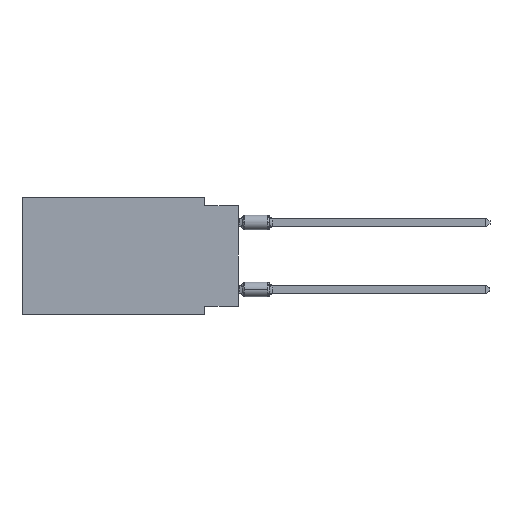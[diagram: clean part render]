
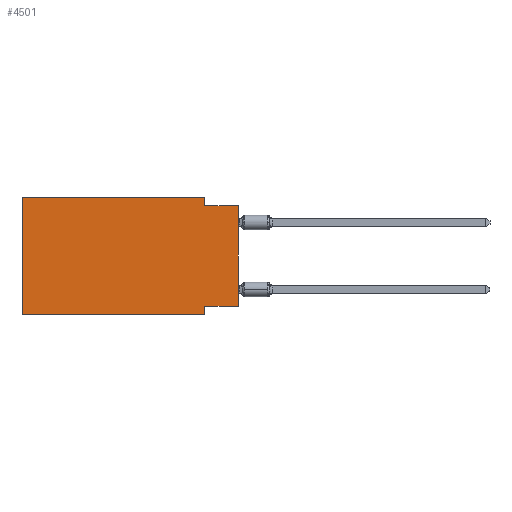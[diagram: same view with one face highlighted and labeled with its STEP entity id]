
A CAD part, left-side view. The second image highlights one B-rep face of the part: STEP entity #4501.
In plain terms, the highlighted planar face has unit normal (-1, 0, 0).
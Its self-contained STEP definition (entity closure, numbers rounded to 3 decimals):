
#44 = VECTOR ( 'NONE', #213, 1000. ) ;
#213 = DIRECTION ( 'NONE',  ( 0., 0., -1. ) ) ;
#262 = DIRECTION ( 'NONE',  ( 0., -1., 0. ) ) ;
#1433 = VECTOR ( 'NONE', #262, 1000. ) ;
#1509 = LINE ( 'NONE', #4698, #1433 ) ;
#1945 = VERTEX_POINT ( 'NONE', #4365 ) ;
#2115 = CARTESIAN_POINT ( 'NONE',  ( 0., 16.383, 0. ) ) ;
#2302 = CARTESIAN_POINT ( 'NONE',  ( 0., 0., -8.255 ) ) ;
#2390 = CARTESIAN_POINT ( 'NONE',  ( 0., 0., -8.255 ) ) ;
#2493 = DIRECTION ( 'NONE',  ( 0., -1., 0. ) ) ;
#2716 = DIRECTION ( 'NONE',  ( 0., 0., -1. ) ) ;
#3091 = DIRECTION ( 'NONE',  ( 0., 0., 1. ) ) ;
#3220 = LINE ( 'NONE', #2390, #13287 ) ;
#3222 = EDGE_CURVE ( 'NONE', #7645, #12915, #7811, .T. ) ;
#3392 = CARTESIAN_POINT ( 'NONE',  ( 0., 16.383, 0. ) ) ;
#3419 = VECTOR ( 'NONE', #2716, 1000. ) ;
#3445 = EDGE_CURVE ( 'NONE', #5342, #11242, #9106, .T. ) ;
#4265 = DIRECTION ( 'NONE',  ( 0., 1., 0. ) ) ;
#4323 = LINE ( 'NONE', #7344, #7355 ) ;
#4365 = CARTESIAN_POINT ( 'NONE',  ( 0., 2.54, 0. ) ) ;
#4501 = ADVANCED_FACE ( 'NONE', ( #11886 ), #9807, .F. ) ;
#4565 = VERTEX_POINT ( 'NONE', #12417 ) ;
#4698 = CARTESIAN_POINT ( 'NONE',  ( 0., 0., -0.635 ) ) ;
#5342 = VERTEX_POINT ( 'NONE', #2302 ) ;
#5819 = EDGE_CURVE ( 'NONE', #5342, #7645, #3220, .T. ) ;
#6143 = ORIENTED_EDGE ( 'NONE', *, *, #3222, .F. ) ;
#6199 = VERTEX_POINT ( 'NONE', #9543 ) ;
#6207 = EDGE_CURVE ( 'NONE', #4565, #12915, #4323, .T. ) ;
#6548 = EDGE_CURVE ( 'NONE', #1945, #13433, #13327, .T. ) ;
#6882 = ORIENTED_EDGE ( 'NONE', *, *, #6207, .T. ) ;
#7131 = EDGE_CURVE ( 'NONE', #13433, #11242, #1509, .T. ) ;
#7344 = CARTESIAN_POINT ( 'NONE',  ( 0., 16.383, -8.89 ) ) ;
#7355 = VECTOR ( 'NONE', #8504, 1000. ) ;
#7645 = VERTEX_POINT ( 'NONE', #11917 ) ;
#7674 = CARTESIAN_POINT ( 'NONE',  ( 0., 16.383, 0. ) ) ;
#7749 = DIRECTION ( 'NONE',  ( 1., 0., 0. ) ) ;
#7811 = LINE ( 'NONE', #11882, #44 ) ;
#8504 = DIRECTION ( 'NONE',  ( 0., -1., 0. ) ) ;
#8755 = EDGE_CURVE ( 'NONE', #4565, #6199, #11571, .T. ) ;
#8764 = DIRECTION ( 'NONE',  ( 0., 0., -1. ) ) ;
#8777 = VECTOR ( 'NONE', #2493, 1000. ) ;
#9106 = LINE ( 'NONE', #10215, #10402 ) ;
#9543 = CARTESIAN_POINT ( 'NONE',  ( 0., 16.383, 0. ) ) ;
#9723 = CARTESIAN_POINT ( 'NONE',  ( 0., 0., -0.635 ) ) ;
#9807 = PLANE ( 'NONE',  #13604 ) ;
#10043 = EDGE_CURVE ( 'NONE', #6199, #1945, #13099, .T. ) ;
#10215 = CARTESIAN_POINT ( 'NONE',  ( 0., 0., 0. ) ) ;
#10366 = CARTESIAN_POINT ( 'NONE',  ( 0., 2.54, 0. ) ) ;
#10402 = VECTOR ( 'NONE', #11111, 1000. ) ;
#10504 = VECTOR ( 'NONE', #3091, 1000. ) ;
#10671 = ORIENTED_EDGE ( 'NONE', *, *, #10043, .F. ) ;
#10714 = ORIENTED_EDGE ( 'NONE', *, *, #3445, .T. ) ;
#11111 = DIRECTION ( 'NONE',  ( 0., 0., 1. ) ) ;
#11242 = VERTEX_POINT ( 'NONE', #9723 ) ;
#11255 = ORIENTED_EDGE ( 'NONE', *, *, #6548, .F. ) ;
#11409 = EDGE_LOOP ( 'NONE', ( #10714, #13311, #11255, #10671, #12628, #6882, #6143, #12290 ) ) ;
#11571 = LINE ( 'NONE', #2115, #10504 ) ;
#11882 = CARTESIAN_POINT ( 'NONE',  ( 0., 2.54, -8.89 ) ) ;
#11886 = FACE_OUTER_BOUND ( 'NONE', #11409, .T. ) ;
#11917 = CARTESIAN_POINT ( 'NONE',  ( 0., 2.54, -8.255 ) ) ;
#12203 = CARTESIAN_POINT ( 'NONE',  ( 0., 2.54, -8.89 ) ) ;
#12290 = ORIENTED_EDGE ( 'NONE', *, *, #5819, .F. ) ;
#12417 = CARTESIAN_POINT ( 'NONE',  ( 0., 16.383, -8.89 ) ) ;
#12628 = ORIENTED_EDGE ( 'NONE', *, *, #8755, .F. ) ;
#12915 = VERTEX_POINT ( 'NONE', #12203 ) ;
#13099 = LINE ( 'NONE', #3392, #8777 ) ;
#13119 = CARTESIAN_POINT ( 'NONE',  ( 0., 2.54, -0.635 ) ) ;
#13287 = VECTOR ( 'NONE', #4265, 1000. ) ;
#13311 = ORIENTED_EDGE ( 'NONE', *, *, #7131, .F. ) ;
#13327 = LINE ( 'NONE', #10366, #3419 ) ;
#13433 = VERTEX_POINT ( 'NONE', #13119 ) ;
#13604 = AXIS2_PLACEMENT_3D ( 'NONE', #7674, #7749, #8764 ) ;
